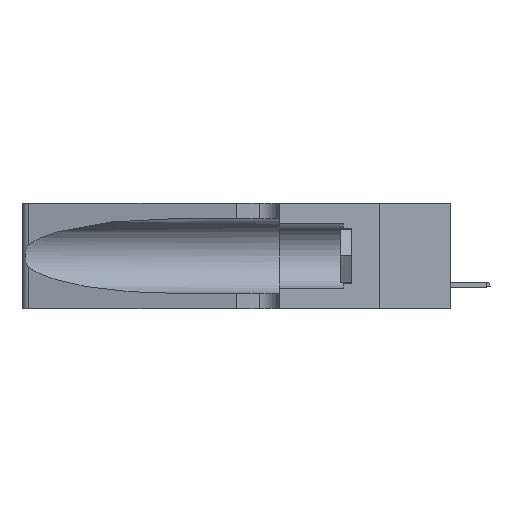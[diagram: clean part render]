
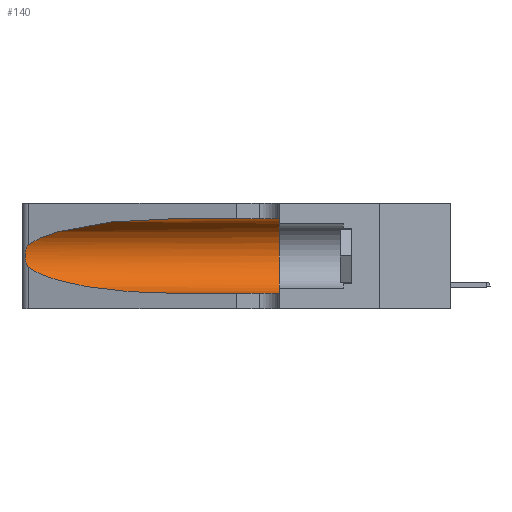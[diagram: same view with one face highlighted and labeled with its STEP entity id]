
A CAD part, left-side view. The second image highlights one B-rep face of the part: STEP entity #140.
In plain terms, the highlighted cylindrical face has radius 3.308 mm (diameter 6.617 mm), a partial arc.
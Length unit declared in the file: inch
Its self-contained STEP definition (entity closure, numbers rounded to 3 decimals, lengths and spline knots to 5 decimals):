
#140 = ADVANCED_FACE ( 'NONE', ( #21894 ), #12969, .F. ) ;
#1805 = AXIS2_PLACEMENT_3D ( 'NONE', #19220, #12849, #32377 ) ;
#2631 = DIRECTION ( 'NONE',  ( 0., -1., 0. ) ) ;
#2636 = ORIENTED_EDGE ( 'NONE', *, *, #19302, .T. ) ;
#3184 = ORIENTED_EDGE ( 'NONE', *, *, #22428, .F. ) ;
#3620 = CARTESIAN_POINT ( 'NONE',  ( 0.1305, 0.72297, 0.05475 ) ) ;
#3879 = ORIENTED_EDGE ( 'NONE', *, *, #39726, .T. ) ;
#4242 = CARTESIAN_POINT ( 'NONE',  ( 0.25856, 1.23593, 0.16098 ) ) ;
#4403 = CARTESIAN_POINT ( 'NONE',  ( 0.1305, 0.72297, 0.31525 ) ) ;
#5441 = EDGE_CURVE ( 'NONE', #21993, #16547, #34719, .T. ) ;
#5495 = ORIENTED_EDGE ( 'NONE', *, *, #40331, .T. ) ;
#6912 = EDGE_LOOP ( 'NONE', ( #5495, #2636, #38939, #3879, #9606, #3184 ) ) ;
#8930 = VECTOR ( 'NONE', #38096, 39.37008 ) ;
#9606 = ORIENTED_EDGE ( 'NONE', *, *, #30368, .F. ) ;
#9771 = CARTESIAN_POINT ( 'NONE',  ( 0.25639, 1.23184, 0.21858 ) ) ;
#9813 = DIRECTION ( 'NONE',  ( 0., 0., -1. ) ) ;
#10183 = CARTESIAN_POINT ( 'NONE',  ( 0.25555, 1.22993, 0.14849 ) ) ;
#12228 = CARTESIAN_POINT ( 'NONE',  ( 0.1305, 0.72297, 0.05475 ) ) ;
#12343 = B_SPLINE_CURVE_WITH_KNOTS ( 'NONE', 3,
 ( #23109, #33267, #9771, #13360, #36452, #26291, #29258, #39656, #39448, #4242, #13143, #16759, #10183, #36041 ),
 .UNSPECIFIED., .F., .F.,
 ( 4, 2, 2, 2, 2, 2, 4 ),
 ( 0., 0.00027, 0.00053, 0.00107, 0.0016, 0.00187, 0.00214 ),
 .UNSPECIFIED. ) ;
#12849 = DIRECTION ( 'NONE',  ( 0., 1., 0. ) ) ;
#12969 = CYLINDRICAL_SURFACE ( 'NONE', #37538, 0.13025 ) ;
#13143 = CARTESIAN_POINT ( 'NONE',  ( 0.25789, 1.23486, 0.15765 ) ) ;
#13360 = CARTESIAN_POINT ( 'NONE',  ( 0.25787, 1.23484, 0.2124 ) ) ;
#14401 =( BOUNDED_CURVE ( )  B_SPLINE_CURVE ( 3, ( #4403, #36805, #23671, #33634 ),
 .UNSPECIFIED., .F., .T. ) 
 B_SPLINE_CURVE_WITH_KNOTS ( ( 4, 4 ),
 ( 1.5708, 2.84003 ),
 .UNSPECIFIED. ) 
 CURVE ( )  GEOMETRIC_REPRESENTATION_ITEM ( )  RATIONAL_B_SPLINE_CURVE ( ( 1., 0.87, 0.87, 1. ) ) 
 REPRESENTATION_ITEM ( '' )  );
#15967 = CARTESIAN_POINT ( 'NONE',  ( 0.1305, 1.61858, 0.05475 ) ) ;
#16063 = CARTESIAN_POINT ( 'NONE',  ( 0.25487, 1.22718, 0.14631 ) ) ;
#16547 = VERTEX_POINT ( 'NONE', #3620 ) ;
#16759 = CARTESIAN_POINT ( 'NONE',  ( 0.25639, 1.23186, 0.15144 ) ) ;
#17881 = VERTEX_POINT ( 'NONE', #29870 ) ;
#19033 = VERTEX_POINT ( 'NONE', #28681 ) ;
#19220 = CARTESIAN_POINT ( 'NONE',  ( 0.1305, 0.35, 0.185 ) ) ;
#19302 = EDGE_CURVE ( 'NONE', #38033, #21993, #12343, .T. ) ;
#21233 = CARTESIAN_POINT ( 'NONE',  ( 0.1305, 0.72297, 0.31525 ) ) ;
#21894 = FACE_OUTER_BOUND ( 'NONE', #6912, .T. ) ;
#21993 = VERTEX_POINT ( 'NONE', #40767 ) ;
#22013 = VERTEX_POINT ( 'NONE', #21233 ) ;
#22428 = EDGE_CURVE ( 'NONE', #22013, #19033, #32152, .T. ) ;
#23109 = CARTESIAN_POINT ( 'NONE',  ( 0.25487, 1.22718, 0.22369 ) ) ;
#23671 = CARTESIAN_POINT ( 'NONE',  ( 0.2373, 1.15595, 0.28018 ) ) ;
#25806 = CARTESIAN_POINT ( 'NONE',  ( 0.2373, 1.15595, 0.08982 ) ) ;
#26138 = LINE ( 'NONE', #15967, #38214 ) ;
#26291 = CARTESIAN_POINT ( 'NONE',  ( 0.26018, 1.23835, 0.19895 ) ) ;
#28543 = CARTESIAN_POINT ( 'NONE',  ( 0.1305, 1.61858, 0.31525 ) ) ;
#28681 = CARTESIAN_POINT ( 'NONE',  ( 0.1305, 0.35, 0.31525 ) ) ;
#29258 = CARTESIAN_POINT ( 'NONE',  ( 0.26075, 1.23896, 0.19203 ) ) ;
#29870 = CARTESIAN_POINT ( 'NONE',  ( 0.1305, 0.35, 0.05475 ) ) ;
#30191 = CIRCLE ( 'NONE', #1805, 0.13025 ) ;
#30368 = EDGE_CURVE ( 'NONE', #19033, #17881, #30191, .T. ) ;
#31655 = CARTESIAN_POINT ( 'NONE',  ( 0.1305, 1.61858, 0.185 ) ) ;
#31668 = DIRECTION ( 'NONE',  ( 0., -1., 0. ) ) ;
#32152 = LINE ( 'NONE', #28543, #8930 ) ;
#32377 = DIRECTION ( 'NONE',  ( 0., 0., 1. ) ) ;
#33267 = CARTESIAN_POINT ( 'NONE',  ( 0.25555, 1.22994, 0.2215 ) ) ;
#33634 = CARTESIAN_POINT ( 'NONE',  ( 0.25487, 1.22718, 0.22369 ) ) ;
#34719 =( BOUNDED_CURVE ( )  B_SPLINE_CURVE ( 3, ( #16063, #25806, #34937, #12228 ),
 .UNSPECIFIED., .F., .T. ) 
 B_SPLINE_CURVE_WITH_KNOTS ( ( 4, 4 ),
 ( 3.44316, 4.71239 ),
 .UNSPECIFIED. ) 
 CURVE ( )  GEOMETRIC_REPRESENTATION_ITEM ( )  RATIONAL_B_SPLINE_CURVE ( ( 1., 0.87, 0.87, 1. ) ) 
 REPRESENTATION_ITEM ( '' )  );
#34937 = CARTESIAN_POINT ( 'NONE',  ( 0.18966, 0.96281, 0.05475 ) ) ;
#36041 = CARTESIAN_POINT ( 'NONE',  ( 0.25487, 1.22718, 0.14631 ) ) ;
#36452 = CARTESIAN_POINT ( 'NONE',  ( 0.25854, 1.2359, 0.20912 ) ) ;
#36805 = CARTESIAN_POINT ( 'NONE',  ( 0.18966, 0.96281, 0.31525 ) ) ;
#37538 = AXIS2_PLACEMENT_3D ( 'NONE', #31655, #2631, #9813 ) ;
#38033 = VERTEX_POINT ( 'NONE', #41874 ) ;
#38096 = DIRECTION ( 'NONE',  ( 0., -1., 0. ) ) ;
#38214 = VECTOR ( 'NONE', #31668, 39.37008 ) ;
#38939 = ORIENTED_EDGE ( 'NONE', *, *, #5441, .T. ) ;
#39448 = CARTESIAN_POINT ( 'NONE',  ( 0.26017, 1.23833, 0.17102 ) ) ;
#39656 = CARTESIAN_POINT ( 'NONE',  ( 0.26075, 1.23896, 0.178 ) ) ;
#39726 = EDGE_CURVE ( 'NONE', #16547, #17881, #26138, .T. ) ;
#40331 = EDGE_CURVE ( 'NONE', #22013, #38033, #14401, .T. ) ;
#40767 = CARTESIAN_POINT ( 'NONE',  ( 0.25487, 1.22718, 0.14631 ) ) ;
#41874 = CARTESIAN_POINT ( 'NONE',  ( 0.25487, 1.22718, 0.22369 ) ) ;
